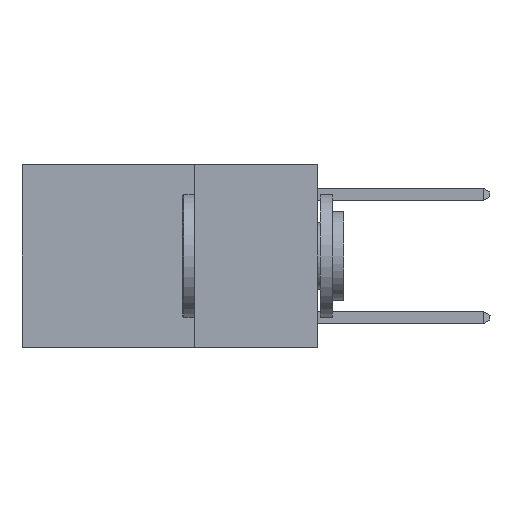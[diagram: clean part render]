
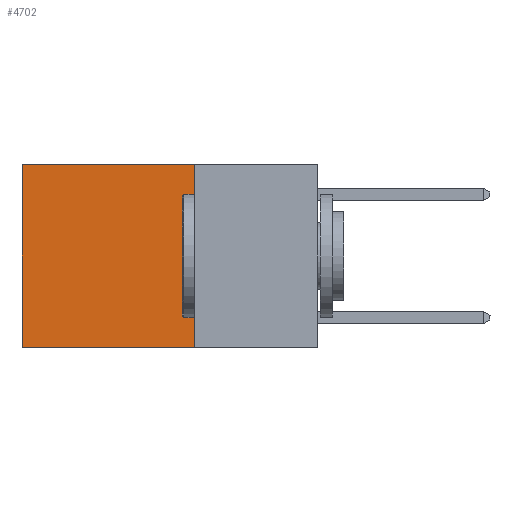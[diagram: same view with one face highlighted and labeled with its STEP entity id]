
A CAD part, left-side view. The second image highlights one B-rep face of the part: STEP entity #4702.
In plain terms, the highlighted planar face has unit normal (-1, 0, 0).
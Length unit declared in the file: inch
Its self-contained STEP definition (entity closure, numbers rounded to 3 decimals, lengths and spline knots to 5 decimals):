
#864 = LINE ( 'NONE', #13904, #25554 ) ;
#1269 = DIRECTION ( 'NONE',  ( 1., 0., 0. ) ) ;
#1695 = EDGE_CURVE ( 'NONE', #27626, #2482, #3899, .T. ) ;
#1824 = ORIENTED_EDGE ( 'NONE', *, *, #1695, .T. ) ;
#2015 = DIRECTION ( 'NONE',  ( 0., 1., 0. ) ) ;
#2482 = VERTEX_POINT ( 'NONE', #5348 ) ;
#3140 = CARTESIAN_POINT ( 'NONE',  ( 0.2625, 0.6, 0. ) ) ;
#3666 = DIRECTION ( 'NONE',  ( 0., 0., -1. ) ) ;
#3899 = LINE ( 'NONE', #25337, #9608 ) ;
#4702 = ADVANCED_FACE ( 'NONE', ( #24348 ), #13387, .F. ) ;
#5300 = AXIS2_PLACEMENT_3D ( 'NONE', #29754, #1269, #18184 ) ;
#5348 = CARTESIAN_POINT ( 'NONE',  ( 0.2625, 0.6, -0.37 ) ) ;
#6032 = CARTESIAN_POINT ( 'NONE',  ( 0.2625, 0.25, 0. ) ) ;
#6561 = EDGE_CURVE ( 'NONE', #14576, #15190, #26410, .T. ) ;
#6876 = VECTOR ( 'NONE', #9459, 39.37008 ) ;
#7027 = CARTESIAN_POINT ( 'NONE',  ( 0.2625, 0.25, -0.37 ) ) ;
#8130 = ORIENTED_EDGE ( 'NONE', *, *, #28728, .T. ) ;
#9139 = LINE ( 'NONE', #7027, #6876 ) ;
#9459 = DIRECTION ( 'NONE',  ( 0., 1., 0. ) ) ;
#9608 = VECTOR ( 'NONE', #13601, 39.37008 ) ;
#13387 = PLANE ( 'NONE',  #5300 ) ;
#13601 = DIRECTION ( 'NONE',  ( 0., 0., -1. ) ) ;
#13904 = CARTESIAN_POINT ( 'NONE',  ( 0.2625, 0.25, 0. ) ) ;
#14229 = ORIENTED_EDGE ( 'NONE', *, *, #6561, .F. ) ;
#14576 = VERTEX_POINT ( 'NONE', #17470 ) ;
#15190 = VERTEX_POINT ( 'NONE', #26535 ) ;
#16963 = EDGE_CURVE ( 'NONE', #15190, #2482, #9139, .T. ) ;
#17470 = CARTESIAN_POINT ( 'NONE',  ( 0.2625, 0.25, 0. ) ) ;
#18184 = DIRECTION ( 'NONE',  ( 0., 0., -1. ) ) ;
#19518 = VECTOR ( 'NONE', #3666, 39.37008 ) ;
#23328 = EDGE_LOOP ( 'NONE', ( #1824, #27084, #14229, #8130 ) ) ;
#24348 = FACE_OUTER_BOUND ( 'NONE', #23328, .T. ) ;
#25337 = CARTESIAN_POINT ( 'NONE',  ( 0.2625, 0.6, 0. ) ) ;
#25554 = VECTOR ( 'NONE', #2015, 39.37008 ) ;
#26410 = LINE ( 'NONE', #6032, #19518 ) ;
#26535 = CARTESIAN_POINT ( 'NONE',  ( 0.2625, 0.25, -0.37 ) ) ;
#27084 = ORIENTED_EDGE ( 'NONE', *, *, #16963, .F. ) ;
#27626 = VERTEX_POINT ( 'NONE', #3140 ) ;
#28728 = EDGE_CURVE ( 'NONE', #14576, #27626, #864, .T. ) ;
#29754 = CARTESIAN_POINT ( 'NONE',  ( 0.2625, 0.25, 0. ) ) ;
